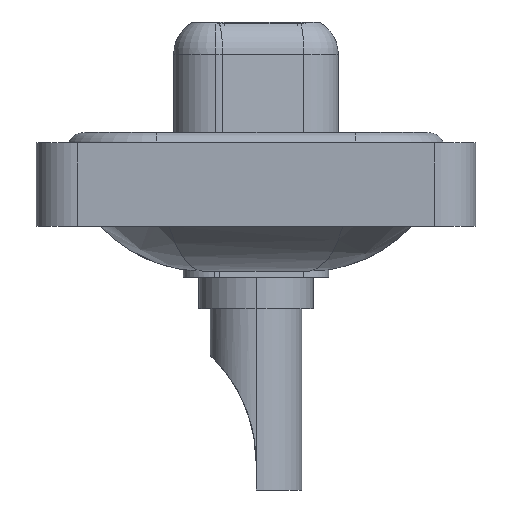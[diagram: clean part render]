
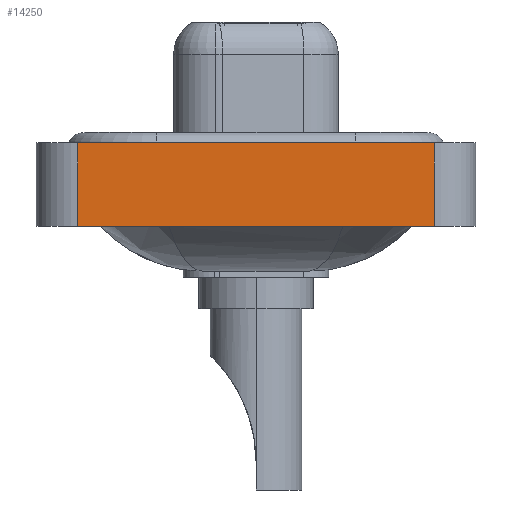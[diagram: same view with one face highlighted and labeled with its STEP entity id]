
A CAD part, left-side view. The second image highlights one B-rep face of the part: STEP entity #14250.
In plain terms, the highlighted planar face has unit normal (-1, 0, 0).
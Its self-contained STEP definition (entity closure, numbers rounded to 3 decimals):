
#1474 = CARTESIAN_POINT ( 'NONE',  ( -7.25, -8.55, -3.6 ) ) ;
#1527 = VERTEX_POINT ( 'NONE', #8513 ) ;
#2407 = CARTESIAN_POINT ( 'NONE',  ( -7.25, -8.55, -3.6 ) ) ;
#3300 = EDGE_CURVE ( 'NONE', #10821, #15981, #14261, .T. ) ;
#3473 = FACE_OUTER_BOUND ( 'NONE', #8629, .T. ) ;
#3559 = DIRECTION ( 'NONE',  ( -1., 0., 0. ) ) ;
#3690 = DIRECTION ( 'NONE',  ( 0., -1., 0. ) ) ;
#4156 = DIRECTION ( 'NONE',  ( 0., 0., 1. ) ) ;
#4852 = CARTESIAN_POINT ( 'NONE',  ( -7.25, -8.55, 0.4 ) ) ;
#4913 = ORIENTED_EDGE ( 'NONE', *, *, #8806, .F. ) ;
#5156 = CARTESIAN_POINT ( 'NONE',  ( -7.25, -8.55, -3.6 ) ) ;
#5310 = VECTOR ( 'NONE', #3690, 1000. ) ;
#5820 = AXIS2_PLACEMENT_3D ( 'NONE', #2407, #3559, #9505 ) ;
#6031 = ORIENTED_EDGE ( 'NONE', *, *, #15838, .F. ) ;
#6726 = DIRECTION ( 'NONE',  ( 0., 0., 1. ) ) ;
#7113 = VECTOR ( 'NONE', #4156, 1000. ) ;
#7248 = ORIENTED_EDGE ( 'NONE', *, *, #13256, .T. ) ;
#7661 = VERTEX_POINT ( 'NONE', #15638 ) ;
#8513 = CARTESIAN_POINT ( 'NONE',  ( -7.25, 8.55, 0.4 ) ) ;
#8629 = EDGE_LOOP ( 'NONE', ( #14002, #4913, #6031, #7248 ) ) ;
#8648 = VECTOR ( 'NONE', #6726, 1000. ) ;
#8806 = EDGE_CURVE ( 'NONE', #1527, #15981, #14948, .T. ) ;
#9315 = CARTESIAN_POINT ( 'NONE',  ( -7.25, 8.55, -3.6 ) ) ;
#9419 = VECTOR ( 'NONE', #10109, 1000. ) ;
#9505 = DIRECTION ( 'NONE',  ( 0., 0., 1. ) ) ;
#10109 = DIRECTION ( 'NONE',  ( 0., -1., 0. ) ) ;
#10821 = VERTEX_POINT ( 'NONE', #12871 ) ;
#11873 = LINE ( 'NONE', #9315, #8648 ) ;
#12871 = CARTESIAN_POINT ( 'NONE',  ( -7.25, -8.55, -3.6 ) ) ;
#13255 = PLANE ( 'NONE',  #5820 ) ;
#13256 = EDGE_CURVE ( 'NONE', #7661, #10821, #15427, .T. ) ;
#13645 = CARTESIAN_POINT ( 'NONE',  ( -7.25, -8.55, 0.4 ) ) ;
#14002 = ORIENTED_EDGE ( 'NONE', *, *, #3300, .T. ) ;
#14250 = ADVANCED_FACE ( 'NONE', ( #3473 ), #13255, .T. ) ;
#14261 = LINE ( 'NONE', #1474, #7113 ) ;
#14948 = LINE ( 'NONE', #13645, #5310 ) ;
#15427 = LINE ( 'NONE', #5156, #9419 ) ;
#15638 = CARTESIAN_POINT ( 'NONE',  ( -7.25, 8.55, -3.6 ) ) ;
#15838 = EDGE_CURVE ( 'NONE', #7661, #1527, #11873, .T. ) ;
#15981 = VERTEX_POINT ( 'NONE', #4852 ) ;
